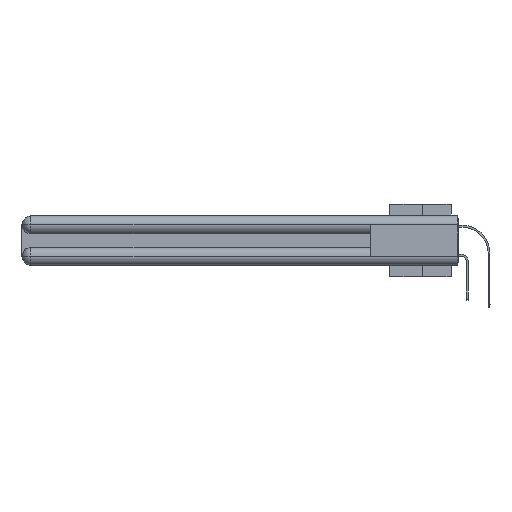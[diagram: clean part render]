
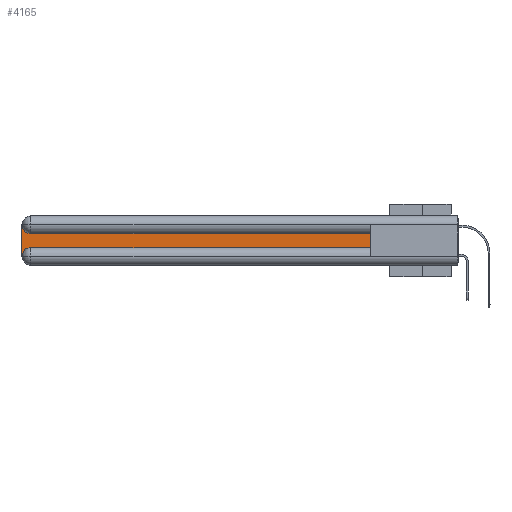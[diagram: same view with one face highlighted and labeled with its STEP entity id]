
A CAD part, left-side view. The second image highlights one B-rep face of the part: STEP entity #4165.
In plain terms, the highlighted planar face has unit normal (-1, 0, 0).
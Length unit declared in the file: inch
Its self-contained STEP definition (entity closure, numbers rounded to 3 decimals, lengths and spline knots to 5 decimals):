
#384 = CARTESIAN_POINT ( 'NONE',  ( 0.075, 0.6, -0.2175 ) ) ;
#1490 = ORIENTED_EDGE ( 'NONE', *, *, #21670, .T. ) ;
#2233 = CARTESIAN_POINT ( 'NONE',  ( 0.075, 3., -0.0625 ) ) ;
#4047 = LINE ( 'NONE', #18410, #8334 ) ;
#4165 = ADVANCED_FACE ( 'NONE', ( #10327 ), #5261, .F. ) ;
#5261 = PLANE ( 'NONE',  #16405 ) ;
#5919 = VERTEX_POINT ( 'NONE', #11985 ) ;
#7249 = VERTEX_POINT ( 'NONE', #384 ) ;
#7865 = CARTESIAN_POINT ( 'NONE',  ( 0.075, 2.94, -0.1225 ) ) ;
#8334 = VECTOR ( 'NONE', #13999, 39.37008 ) ;
#8532 = ORIENTED_EDGE ( 'NONE', *, *, #18500, .T. ) ;
#9752 = CIRCLE ( 'NONE', #20705, 0.06 ) ;
#10327 = FACE_OUTER_BOUND ( 'NONE', #30727, .T. ) ;
#10488 = DIRECTION ( 'NONE',  ( 0., 0., -1. ) ) ;
#11150 = LINE ( 'NONE', #16211, #32229 ) ;
#11985 = CARTESIAN_POINT ( 'NONE',  ( 0.075, 2.94, -0.2175 ) ) ;
#12247 = EDGE_CURVE ( 'NONE', #28955, #12759, #13172, .T. ) ;
#12666 = ORIENTED_EDGE ( 'NONE', *, *, #27997, .T. ) ;
#12759 = VERTEX_POINT ( 'NONE', #7865 ) ;
#12832 = CIRCLE ( 'NONE', #30576, 0.06 ) ;
#13054 = VERTEX_POINT ( 'NONE', #31363 ) ;
#13172 = LINE ( 'NONE', #18058, #13726 ) ;
#13223 = DIRECTION ( 'NONE',  ( 0., 0., -1. ) ) ;
#13726 = VECTOR ( 'NONE', #28028, 39.37008 ) ;
#13999 = DIRECTION ( 'NONE',  ( 0., 0., 1. ) ) ;
#15484 = DIRECTION ( 'NONE',  ( 0., 0., -1. ) ) ;
#16211 = CARTESIAN_POINT ( 'NONE',  ( 0.075, 3., -0.2175 ) ) ;
#16405 = AXIS2_PLACEMENT_3D ( 'NONE', #27643, #25191, #10488 ) ;
#17675 = ORIENTED_EDGE ( 'NONE', *, *, #12247, .T. ) ;
#18055 = LINE ( 'NONE', #25091, #27478 ) ;
#18058 = CARTESIAN_POINT ( 'NONE',  ( 0.075, 0.6, -0.1225 ) ) ;
#18410 = CARTESIAN_POINT ( 'NONE',  ( 0.075, 0.6, -0.2175 ) ) ;
#18500 = EDGE_CURVE ( 'NONE', #12759, #21571, #12832, .T. ) ;
#20705 = AXIS2_PLACEMENT_3D ( 'NONE', #22663, #22494, #15484 ) ;
#20714 = DIRECTION ( 'NONE',  ( 1., 0., 0. ) ) ;
#21571 = VERTEX_POINT ( 'NONE', #2233 ) ;
#21670 = EDGE_CURVE ( 'NONE', #5919, #7249, #18055, .T. ) ;
#22494 = DIRECTION ( 'NONE',  ( 1., 0., 0. ) ) ;
#22663 = CARTESIAN_POINT ( 'NONE',  ( 0.075, 2.94, -0.2775 ) ) ;
#23887 = DIRECTION ( 'NONE',  ( 0., 0., -1. ) ) ;
#25091 = CARTESIAN_POINT ( 'NONE',  ( 0.075, 0.6, -0.2175 ) ) ;
#25191 = DIRECTION ( 'NONE',  ( 1., 0., 0. ) ) ;
#25731 = EDGE_CURVE ( 'NONE', #13054, #5919, #9752, .T. ) ;
#27478 = VECTOR ( 'NONE', #28026, 39.37008 ) ;
#27643 = CARTESIAN_POINT ( 'NONE',  ( 0.075, 3., -0.1225 ) ) ;
#27997 = EDGE_CURVE ( 'NONE', #21571, #13054, #11150, .T. ) ;
#28026 = DIRECTION ( 'NONE',  ( 0., -1., 0. ) ) ;
#28028 = DIRECTION ( 'NONE',  ( 0., 1., 0. ) ) ;
#28116 = ORIENTED_EDGE ( 'NONE', *, *, #32151, .T. ) ;
#28955 = VERTEX_POINT ( 'NONE', #30132 ) ;
#30132 = CARTESIAN_POINT ( 'NONE',  ( 0.075, 0.6, -0.1225 ) ) ;
#30576 = AXIS2_PLACEMENT_3D ( 'NONE', #31171, #20714, #13223 ) ;
#30727 = EDGE_LOOP ( 'NONE', ( #17675, #8532, #12666, #31455, #1490, #28116 ) ) ;
#31171 = CARTESIAN_POINT ( 'NONE',  ( 0.075, 2.94, -0.0625 ) ) ;
#31363 = CARTESIAN_POINT ( 'NONE',  ( 0.075, 3., -0.2775 ) ) ;
#31455 = ORIENTED_EDGE ( 'NONE', *, *, #25731, .T. ) ;
#32151 = EDGE_CURVE ( 'NONE', #7249, #28955, #4047, .T. ) ;
#32229 = VECTOR ( 'NONE', #23887, 39.37008 ) ;
